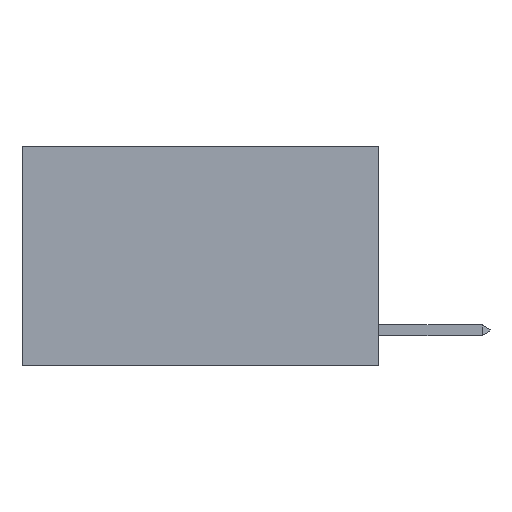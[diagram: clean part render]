
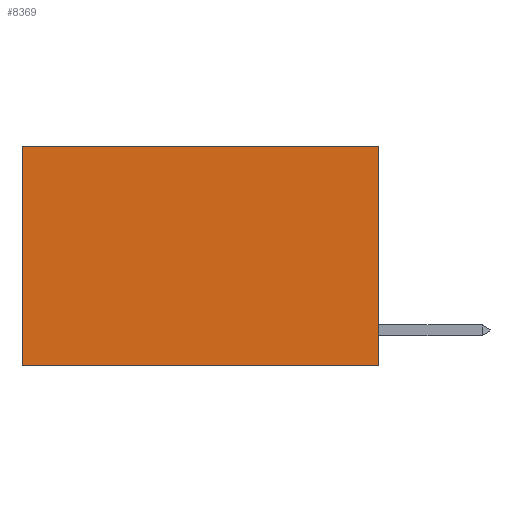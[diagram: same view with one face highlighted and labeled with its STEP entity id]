
A CAD part, left-side view. The second image highlights one B-rep face of the part: STEP entity #8369.
In plain terms, the highlighted planar face has unit normal (-1, 0, 0).
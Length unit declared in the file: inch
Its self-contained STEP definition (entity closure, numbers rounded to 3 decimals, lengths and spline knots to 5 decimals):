
#488 = VERTEX_POINT ( 'NONE', #4854 ) ;
#683 = CARTESIAN_POINT ( 'NONE',  ( 0.2625, 0., 0. ) ) ;
#1658 = CARTESIAN_POINT ( 'NONE',  ( 0.2625, 0., 0. ) ) ;
#2184 = CARTESIAN_POINT ( 'NONE',  ( 0.2625, 0., 0. ) ) ;
#2367 = CARTESIAN_POINT ( 'NONE',  ( 0.2625, 0.6, 0. ) ) ;
#2595 = LINE ( 'NONE', #9692, #13916 ) ;
#2930 = DIRECTION ( 'NONE',  ( 0., 0., -1. ) ) ;
#3302 = DIRECTION ( 'NONE',  ( 0., 0., -1. ) ) ;
#3409 = CARTESIAN_POINT ( 'NONE',  ( 0.2625, 0., 0. ) ) ;
#3483 = LINE ( 'NONE', #1658, #6127 ) ;
#3723 = LINE ( 'NONE', #10881, #6361 ) ;
#4180 = AXIS2_PLACEMENT_3D ( 'NONE', #2184, #9989, #3302 ) ;
#4373 = EDGE_CURVE ( 'NONE', #4687, #488, #2595, .T. ) ;
#4495 = ORIENTED_EDGE ( 'NONE', *, *, #7227, .T. ) ;
#4687 = VERTEX_POINT ( 'NONE', #2367 ) ;
#4854 = CARTESIAN_POINT ( 'NONE',  ( 0.2625, 0.6, -0.37 ) ) ;
#4917 = CARTESIAN_POINT ( 'NONE',  ( 0.2625, 0., -0.37 ) ) ;
#5257 = DIRECTION ( 'NONE',  ( 0., 0., -1. ) ) ;
#5331 = VECTOR ( 'NONE', #2930, 39.37008 ) ;
#6127 = VECTOR ( 'NONE', #7219, 39.37008 ) ;
#6361 = VECTOR ( 'NONE', #14070, 39.37008 ) ;
#7185 = VERTEX_POINT ( 'NONE', #4917 ) ;
#7219 = DIRECTION ( 'NONE',  ( 0., 1., 0. ) ) ;
#7227 = EDGE_CURVE ( 'NONE', #8463, #4687, #3483, .T. ) ;
#8369 = ADVANCED_FACE ( 'NONE', ( #11273 ), #14227, .F. ) ;
#8463 = VERTEX_POINT ( 'NONE', #3409 ) ;
#9313 = ORIENTED_EDGE ( 'NONE', *, *, #4373, .T. ) ;
#9692 = CARTESIAN_POINT ( 'NONE',  ( 0.2625, 0.6, 0. ) ) ;
#9989 = DIRECTION ( 'NONE',  ( 1., 0., 0. ) ) ;
#10881 = CARTESIAN_POINT ( 'NONE',  ( 0.2625, 0., -0.37 ) ) ;
#11246 = LINE ( 'NONE', #683, #5331 ) ;
#11273 = FACE_OUTER_BOUND ( 'NONE', #11335, .T. ) ;
#11335 = EDGE_LOOP ( 'NONE', ( #9313, #13733, #14231, #4495 ) ) ;
#12243 = EDGE_CURVE ( 'NONE', #8463, #7185, #11246, .T. ) ;
#13507 = EDGE_CURVE ( 'NONE', #7185, #488, #3723, .T. ) ;
#13733 = ORIENTED_EDGE ( 'NONE', *, *, #13507, .F. ) ;
#13916 = VECTOR ( 'NONE', #5257, 39.37008 ) ;
#14070 = DIRECTION ( 'NONE',  ( 0., 1., 0. ) ) ;
#14227 = PLANE ( 'NONE',  #4180 ) ;
#14231 = ORIENTED_EDGE ( 'NONE', *, *, #12243, .F. ) ;
